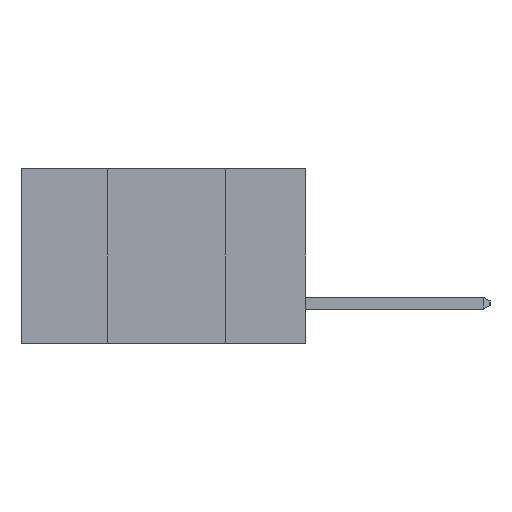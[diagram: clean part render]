
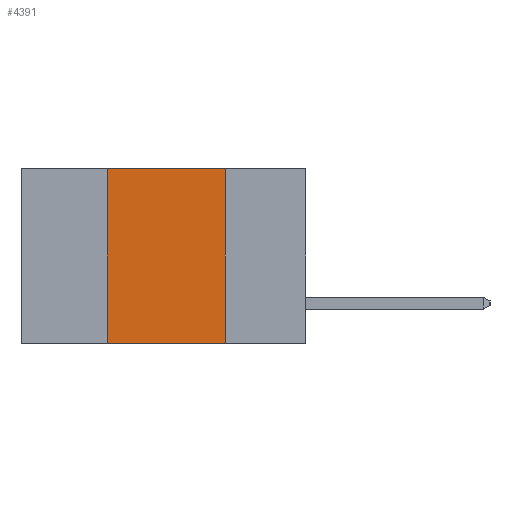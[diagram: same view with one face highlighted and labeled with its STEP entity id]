
A CAD part, left-side view. The second image highlights one B-rep face of the part: STEP entity #4391.
In plain terms, the highlighted planar face has unit normal (-1, 0, 0).
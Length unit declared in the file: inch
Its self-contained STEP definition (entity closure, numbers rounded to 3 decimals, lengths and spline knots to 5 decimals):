
#593 = CARTESIAN_POINT ( 'NONE',  ( 0., 0.6, 0. ) ) ;
#2569 = DIRECTION ( 'NONE',  ( 0., -1., 0. ) ) ;
#3554 = ORIENTED_EDGE ( 'NONE', *, *, #14424, .T. ) ;
#3647 = DIRECTION ( 'NONE',  ( 0., -1., 0. ) ) ;
#4056 = VECTOR ( 'NONE', #18387, 39.37008 ) ;
#4391 = ADVANCED_FACE ( 'NONE', ( #22539 ), #7506, .F. ) ;
#5582 = CARTESIAN_POINT ( 'NONE',  ( 0., 0.6, -0.37 ) ) ;
#6074 = EDGE_CURVE ( 'NONE', #9719, #23292, #13250, .T. ) ;
#6903 = EDGE_CURVE ( 'NONE', #23549, #17486, #8649, .T. ) ;
#7347 = DIRECTION ( 'NONE',  ( 0., 0., -1. ) ) ;
#7369 = DIRECTION ( 'NONE',  ( 1., 0., 0. ) ) ;
#7506 = PLANE ( 'NONE',  #16707 ) ;
#7680 = CARTESIAN_POINT ( 'NONE',  ( 0., 0.6, 0. ) ) ;
#8649 = LINE ( 'NONE', #18437, #4056 ) ;
#8748 = DIRECTION ( 'NONE',  ( 0., 0., 1. ) ) ;
#9518 = CARTESIAN_POINT ( 'NONE',  ( 0., 0.42, 0. ) ) ;
#9664 = CARTESIAN_POINT ( 'NONE',  ( 0., 0.17, -0.37 ) ) ;
#9719 = VERTEX_POINT ( 'NONE', #10448 ) ;
#10182 = LINE ( 'NONE', #5582, #25018 ) ;
#10448 = CARTESIAN_POINT ( 'NONE',  ( 0., 0.42, -0.37 ) ) ;
#11800 = ORIENTED_EDGE ( 'NONE', *, *, #6903, .F. ) ;
#13250 = LINE ( 'NONE', #9518, #22969 ) ;
#14020 = EDGE_CURVE ( 'NONE', #23292, #23549, #14745, .T. ) ;
#14424 = EDGE_CURVE ( 'NONE', #9719, #17486, #10182, .T. ) ;
#14595 = CARTESIAN_POINT ( 'NONE',  ( 0., 0.17, 0. ) ) ;
#14745 = LINE ( 'NONE', #593, #24445 ) ;
#14758 = EDGE_LOOP ( 'NONE', ( #11800, #24536, #20639, #3554 ) ) ;
#16707 = AXIS2_PLACEMENT_3D ( 'NONE', #7680, #7369, #7347 ) ;
#17486 = VERTEX_POINT ( 'NONE', #9664 ) ;
#18387 = DIRECTION ( 'NONE',  ( 0., 0., -1. ) ) ;
#18437 = CARTESIAN_POINT ( 'NONE',  ( 0., 0.17, 0. ) ) ;
#20639 = ORIENTED_EDGE ( 'NONE', *, *, #6074, .F. ) ;
#22539 = FACE_OUTER_BOUND ( 'NONE', #14758, .T. ) ;
#22969 = VECTOR ( 'NONE', #8748, 39.37008 ) ;
#23292 = VERTEX_POINT ( 'NONE', #23491 ) ;
#23491 = CARTESIAN_POINT ( 'NONE',  ( 0., 0.42, 0. ) ) ;
#23549 = VERTEX_POINT ( 'NONE', #14595 ) ;
#24445 = VECTOR ( 'NONE', #2569, 39.37008 ) ;
#24536 = ORIENTED_EDGE ( 'NONE', *, *, #14020, .F. ) ;
#25018 = VECTOR ( 'NONE', #3647, 39.37008 ) ;
